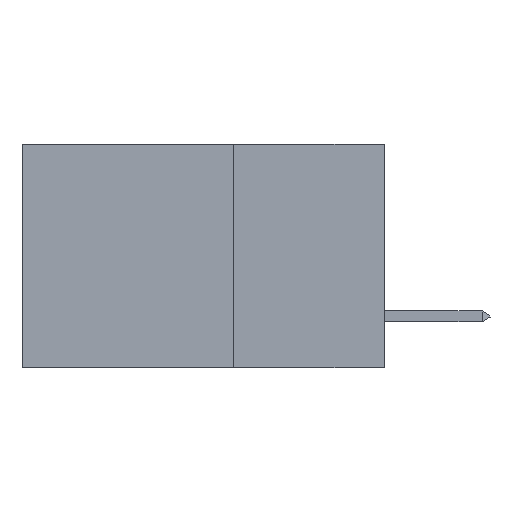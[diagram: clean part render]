
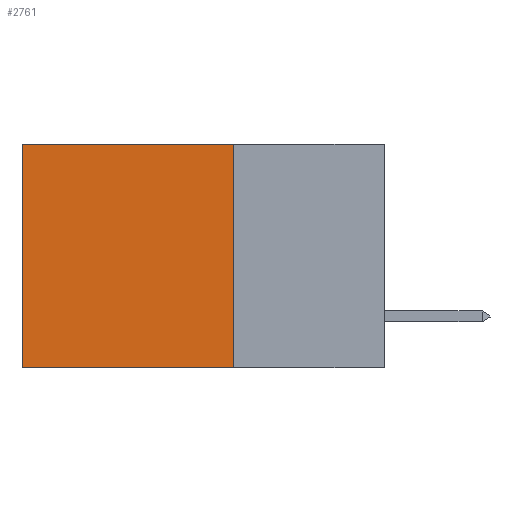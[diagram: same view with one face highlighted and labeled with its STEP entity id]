
A CAD part, left-side view. The second image highlights one B-rep face of the part: STEP entity #2761.
In plain terms, the highlighted planar face has unit normal (-1, 0, 0).
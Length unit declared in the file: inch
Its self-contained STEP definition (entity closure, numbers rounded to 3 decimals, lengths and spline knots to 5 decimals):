
#52 = EDGE_CURVE ( 'NONE', #6175, #5134, #1693, .T. ) ;
#182 = ORIENTED_EDGE ( 'NONE', *, *, #3437, .T. ) ;
#364 = VECTOR ( 'NONE', #6540, 39.37008 ) ;
#628 = EDGE_LOOP ( 'NONE', ( #182, #7677, #3941, #6935 ) ) ;
#967 = DIRECTION ( 'NONE',  ( 0., 0., -1. ) ) ;
#1407 = PLANE ( 'NONE',  #8900 ) ;
#1520 = FACE_OUTER_BOUND ( 'NONE', #628, .T. ) ;
#1588 = DIRECTION ( 'NONE',  ( 0., 0., -1. ) ) ;
#1693 = LINE ( 'NONE', #6719, #5324 ) ;
#2162 = CARTESIAN_POINT ( 'NONE',  ( 0.2875, 0.25, -0.37 ) ) ;
#2761 = ADVANCED_FACE ( 'NONE', ( #1520 ), #1407, .F. ) ;
#3437 = EDGE_CURVE ( 'NONE', #8857, #7637, #7094, .T. ) ;
#3922 = EDGE_CURVE ( 'NONE', #6175, #8857, #6681, .T. ) ;
#3941 = ORIENTED_EDGE ( 'NONE', *, *, #52, .F. ) ;
#3965 = VECTOR ( 'NONE', #8553, 39.37008 ) ;
#4185 = VECTOR ( 'NONE', #5663, 39.37008 ) ;
#5134 = VERTEX_POINT ( 'NONE', #2162 ) ;
#5324 = VECTOR ( 'NONE', #967, 39.37008 ) ;
#5663 = DIRECTION ( 'NONE',  ( 0., 1., 0. ) ) ;
#5798 = CARTESIAN_POINT ( 'NONE',  ( 0.2875, 0.25, 0. ) ) ;
#6175 = VERTEX_POINT ( 'NONE', #8803 ) ;
#6225 = CARTESIAN_POINT ( 'NONE',  ( 0.2875, 0.6, 0. ) ) ;
#6540 = DIRECTION ( 'NONE',  ( 0., 1., 0. ) ) ;
#6681 = LINE ( 'NONE', #5798, #364 ) ;
#6719 = CARTESIAN_POINT ( 'NONE',  ( 0.2875, 0.25, 0. ) ) ;
#6935 = ORIENTED_EDGE ( 'NONE', *, *, #3922, .T. ) ;
#7094 = LINE ( 'NONE', #8665, #3965 ) ;
#7500 = EDGE_CURVE ( 'NONE', #5134, #7637, #9401, .T. ) ;
#7637 = VERTEX_POINT ( 'NONE', #9780 ) ;
#7677 = ORIENTED_EDGE ( 'NONE', *, *, #7500, .F. ) ;
#8200 = CARTESIAN_POINT ( 'NONE',  ( 0.2875, 0.25, -0.37 ) ) ;
#8553 = DIRECTION ( 'NONE',  ( 0., 0., -1. ) ) ;
#8665 = CARTESIAN_POINT ( 'NONE',  ( 0.2875, 0.6, 0. ) ) ;
#8803 = CARTESIAN_POINT ( 'NONE',  ( 0.2875, 0.25, 0. ) ) ;
#8857 = VERTEX_POINT ( 'NONE', #6225 ) ;
#8900 = AXIS2_PLACEMENT_3D ( 'NONE', #9277, #9561, #1588 ) ;
#9277 = CARTESIAN_POINT ( 'NONE',  ( 0.2875, 0.25, 0. ) ) ;
#9401 = LINE ( 'NONE', #8200, #4185 ) ;
#9561 = DIRECTION ( 'NONE',  ( 1., 0., 0. ) ) ;
#9780 = CARTESIAN_POINT ( 'NONE',  ( 0.2875, 0.6, -0.37 ) ) ;
